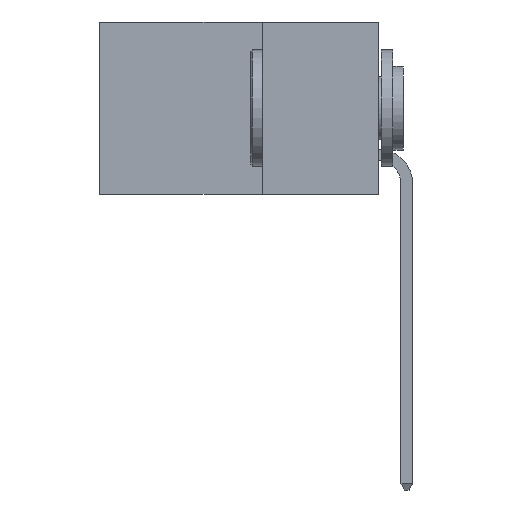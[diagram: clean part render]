
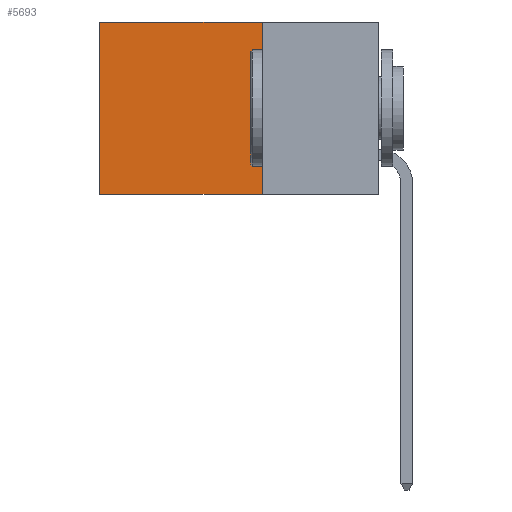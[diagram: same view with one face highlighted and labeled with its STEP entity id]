
A CAD part, left-side view. The second image highlights one B-rep face of the part: STEP entity #5693.
In plain terms, the highlighted planar face has unit normal (-1, 0, 0).
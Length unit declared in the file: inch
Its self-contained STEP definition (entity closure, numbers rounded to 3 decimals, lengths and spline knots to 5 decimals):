
#756 = LINE ( 'NONE', #3850, #7636 ) ;
#1989 = LINE ( 'NONE', #3802, #12323 ) ;
#2393 = FACE_OUTER_BOUND ( 'NONE', #3501, .T. ) ;
#2964 = EDGE_CURVE ( 'NONE', #8166, #13221, #16309, .T. ) ;
#3501 = EDGE_LOOP ( 'NONE', ( #9987, #14240, #5265, #6293 ) ) ;
#3802 = CARTESIAN_POINT ( 'NONE',  ( 0.2615, 0.6, -0.37 ) ) ;
#3850 = CARTESIAN_POINT ( 'NONE',  ( 0.2615, 0.25, -0.37 ) ) ;
#4286 = DIRECTION ( 'NONE',  ( 0., 0., -1. ) ) ;
#4653 = CARTESIAN_POINT ( 'NONE',  ( 0.2615, 0.25, -0.37 ) ) ;
#5265 = ORIENTED_EDGE ( 'NONE', *, *, #2964, .F. ) ;
#5268 = DIRECTION ( 'NONE',  ( 0., 1., 0. ) ) ;
#5693 = ADVANCED_FACE ( 'NONE', ( #2393 ), #5733, .F. ) ;
#5733 = PLANE ( 'NONE',  #12825 ) ;
#5888 = CARTESIAN_POINT ( 'NONE',  ( 0.2615, 0.25, 0. ) ) ;
#5904 = VECTOR ( 'NONE', #4286, 39.37008 ) ;
#6293 = ORIENTED_EDGE ( 'NONE', *, *, #9648, .T. ) ;
#6543 = DIRECTION ( 'NONE',  ( 0., 0., -1. ) ) ;
#7044 = DIRECTION ( 'NONE',  ( 1., 0., 0. ) ) ;
#7636 = VECTOR ( 'NONE', #5268, 39.37008 ) ;
#8166 = VERTEX_POINT ( 'NONE', #14787 ) ;
#9373 = VECTOR ( 'NONE', #13794, 39.37008 ) ;
#9648 = EDGE_CURVE ( 'NONE', #8166, #15766, #15810, .T. ) ;
#9987 = ORIENTED_EDGE ( 'NONE', *, *, #13227, .T. ) ;
#12191 = CARTESIAN_POINT ( 'NONE',  ( 0.2615, 0.6, 0. ) ) ;
#12323 = VECTOR ( 'NONE', #6543, 39.37008 ) ;
#12825 = AXIS2_PLACEMENT_3D ( 'NONE', #14920, #7044, #16174 ) ;
#13148 = CARTESIAN_POINT ( 'NONE',  ( 0.2615, 0.25, -0.37 ) ) ;
#13221 = VERTEX_POINT ( 'NONE', #13148 ) ;
#13227 = EDGE_CURVE ( 'NONE', #15766, #13978, #1989, .T. ) ;
#13794 = DIRECTION ( 'NONE',  ( 0., 1., 0. ) ) ;
#13978 = VERTEX_POINT ( 'NONE', #17245 ) ;
#14240 = ORIENTED_EDGE ( 'NONE', *, *, #15837, .F. ) ;
#14787 = CARTESIAN_POINT ( 'NONE',  ( 0.2615, 0.25, 0. ) ) ;
#14920 = CARTESIAN_POINT ( 'NONE',  ( 0.2615, 0.25, -0.37 ) ) ;
#15766 = VERTEX_POINT ( 'NONE', #12191 ) ;
#15810 = LINE ( 'NONE', #5888, #9373 ) ;
#15837 = EDGE_CURVE ( 'NONE', #13221, #13978, #756, .T. ) ;
#16174 = DIRECTION ( 'NONE',  ( 0., 0., -1. ) ) ;
#16309 = LINE ( 'NONE', #4653, #5904 ) ;
#17245 = CARTESIAN_POINT ( 'NONE',  ( 0.2615, 0.6, -0.37 ) ) ;
